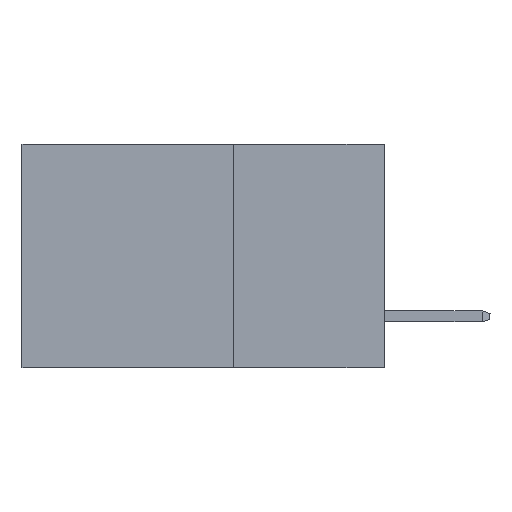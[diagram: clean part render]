
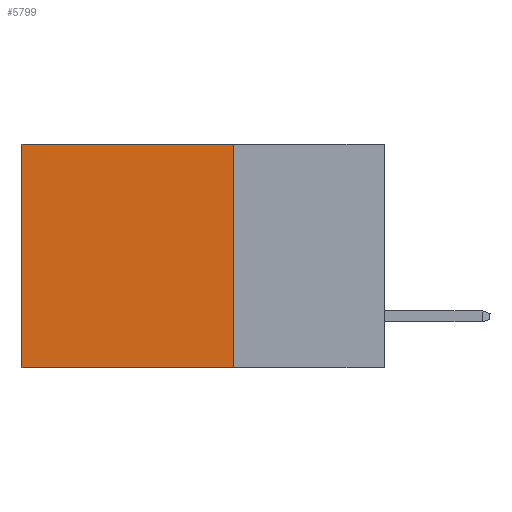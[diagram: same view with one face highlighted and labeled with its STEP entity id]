
A CAD part, left-side view. The second image highlights one B-rep face of the part: STEP entity #5799.
In plain terms, the highlighted planar face has unit normal (-1, 0, 0).
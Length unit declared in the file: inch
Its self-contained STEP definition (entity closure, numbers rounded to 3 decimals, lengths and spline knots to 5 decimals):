
#310 = LINE ( 'NONE', #5668, #3841 ) ;
#464 = DIRECTION ( 'NONE',  ( 0., 1., 0. ) ) ;
#708 = DIRECTION ( 'NONE',  ( 1., 0., 0. ) ) ;
#1854 = CARTESIAN_POINT ( 'NONE',  ( 0.2615, 0.25, -0.37 ) ) ;
#2074 = CARTESIAN_POINT ( 'NONE',  ( 0.2615, 0.25, 0. ) ) ;
#2449 = EDGE_LOOP ( 'NONE', ( #6902, #3108, #8629, #2674 ) ) ;
#2493 = EDGE_CURVE ( 'NONE', #10527, #13239, #5742, .T. ) ;
#2674 = ORIENTED_EDGE ( 'NONE', *, *, #3885, .T. ) ;
#2754 = CARTESIAN_POINT ( 'NONE',  ( 0.2615, 0.6, 0. ) ) ;
#2895 = PLANE ( 'NONE',  #3019 ) ;
#3019 = AXIS2_PLACEMENT_3D ( 'NONE', #1854, #708, #10302 ) ;
#3108 = ORIENTED_EDGE ( 'NONE', *, *, #2493, .F. ) ;
#3841 = VECTOR ( 'NONE', #6730, 39.37008 ) ;
#3885 = EDGE_CURVE ( 'NONE', #11668, #8538, #310, .T. ) ;
#5088 = VECTOR ( 'NONE', #11154, 39.37008 ) ;
#5150 = LINE ( 'NONE', #5902, #5088 ) ;
#5668 = CARTESIAN_POINT ( 'NONE',  ( 0.2615, 0.25, 0. ) ) ;
#5742 = LINE ( 'NONE', #10764, #10882 ) ;
#5799 = ADVANCED_FACE ( 'NONE', ( #8169 ), #2895, .F. ) ;
#5902 = CARTESIAN_POINT ( 'NONE',  ( 0.2615, 0.6, -0.37 ) ) ;
#6464 = CARTESIAN_POINT ( 'NONE',  ( 0.2615, 0.25, -0.37 ) ) ;
#6730 = DIRECTION ( 'NONE',  ( 0., 1., 0. ) ) ;
#6902 = ORIENTED_EDGE ( 'NONE', *, *, #7274, .T. ) ;
#7274 = EDGE_CURVE ( 'NONE', #8538, #13239, #5150, .T. ) ;
#8169 = FACE_OUTER_BOUND ( 'NONE', #2449, .T. ) ;
#8355 = VECTOR ( 'NONE', #10749, 39.37008 ) ;
#8538 = VERTEX_POINT ( 'NONE', #2754 ) ;
#8629 = ORIENTED_EDGE ( 'NONE', *, *, #12621, .F. ) ;
#10302 = DIRECTION ( 'NONE',  ( 0., 0., -1. ) ) ;
#10527 = VERTEX_POINT ( 'NONE', #12677 ) ;
#10684 = LINE ( 'NONE', #6464, #8355 ) ;
#10749 = DIRECTION ( 'NONE',  ( 0., 0., -1. ) ) ;
#10764 = CARTESIAN_POINT ( 'NONE',  ( 0.2615, 0.25, -0.37 ) ) ;
#10882 = VECTOR ( 'NONE', #464, 39.37008 ) ;
#11154 = DIRECTION ( 'NONE',  ( 0., 0., -1. ) ) ;
#11668 = VERTEX_POINT ( 'NONE', #2074 ) ;
#12109 = CARTESIAN_POINT ( 'NONE',  ( 0.2615, 0.6, -0.37 ) ) ;
#12621 = EDGE_CURVE ( 'NONE', #11668, #10527, #10684, .T. ) ;
#12677 = CARTESIAN_POINT ( 'NONE',  ( 0.2615, 0.25, -0.37 ) ) ;
#13239 = VERTEX_POINT ( 'NONE', #12109 ) ;
